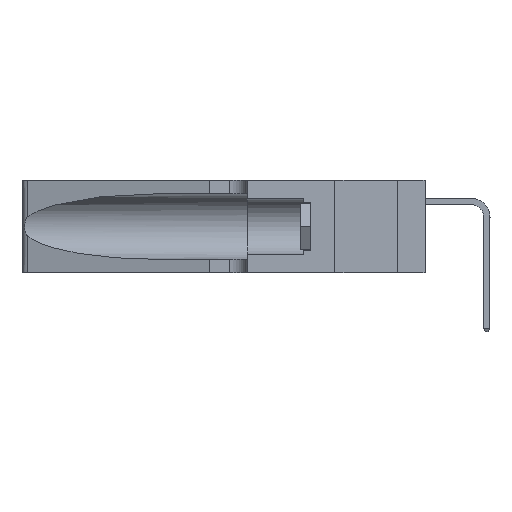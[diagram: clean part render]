
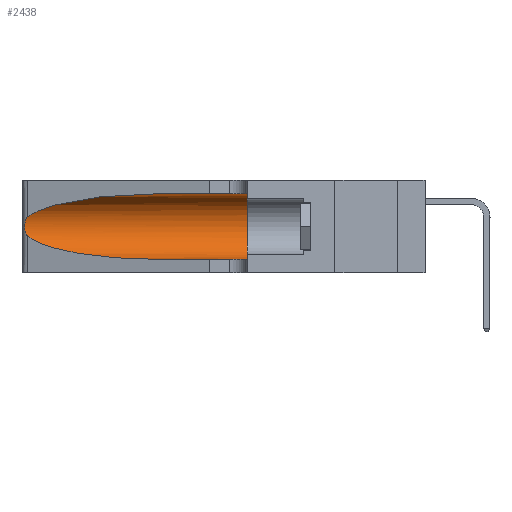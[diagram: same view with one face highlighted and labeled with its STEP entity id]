
A CAD part, left-side view. The second image highlights one B-rep face of the part: STEP entity #2438.
In plain terms, the highlighted cylindrical face has radius 3.308 mm (diameter 6.617 mm), a partial arc.
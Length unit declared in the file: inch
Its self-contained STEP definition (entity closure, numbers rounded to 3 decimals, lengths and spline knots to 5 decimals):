
#8 = CARTESIAN_POINT ( 'NONE',  ( 0.25854, 1.2359, 0.20912 ) ) ;
#1064 = CARTESIAN_POINT ( 'NONE',  ( 0.2373, 1.15595, 0.08982 ) ) ;
#1563 = AXIS2_PLACEMENT_3D ( 'NONE', #12583, #29313, #32099 ) ;
#2438 = ADVANCED_FACE ( 'NONE', ( #8639 ), #29799, .F. ) ;
#2806 = CARTESIAN_POINT ( 'NONE',  ( 0.26075, 1.23896, 0.19203 ) ) ;
#3381 = VERTEX_POINT ( 'NONE', #5818 ) ;
#3689 =( BOUNDED_CURVE ( )  B_SPLINE_CURVE ( 3, ( #4018, #1064, #9629, #28894 ),
 .UNSPECIFIED., .F., .T. ) 
 B_SPLINE_CURVE_WITH_KNOTS ( ( 4, 4 ),
 ( 3.44316, 4.71239 ),
 .UNSPECIFIED. ) 
 CURVE ( )  GEOMETRIC_REPRESENTATION_ITEM ( )  RATIONAL_B_SPLINE_CURVE ( ( 1., 0.87, 0.87, 1. ) ) 
 REPRESENTATION_ITEM ( '' )  );
#4018 = CARTESIAN_POINT ( 'NONE',  ( 0.25487, 1.22718, 0.14631 ) ) ;
#4742 = CARTESIAN_POINT ( 'NONE',  ( 0.1305, 1.61858, 0.05475 ) ) ;
#4888 = DIRECTION ( 'NONE',  ( 0., 1., 0. ) ) ;
#5633 = CARTESIAN_POINT ( 'NONE',  ( 0.26017, 1.23833, 0.17102 ) ) ;
#5818 = CARTESIAN_POINT ( 'NONE',  ( 0.1305, 0.72297, 0.05475 ) ) ;
#6177 = EDGE_CURVE ( 'NONE', #21253, #7064, #14655, .T. ) ;
#7064 = VERTEX_POINT ( 'NONE', #15057 ) ;
#7546 = DIRECTION ( 'NONE',  ( 0., -1., 0. ) ) ;
#7639 =( BOUNDED_CURVE ( )  B_SPLINE_CURVE ( 3, ( #24310, #21574, #27076, #10600 ),
 .UNSPECIFIED., .F., .F. ) 
 B_SPLINE_CURVE_WITH_KNOTS ( ( 4, 4 ),
 ( 1.5708, 2.84003 ),
 .UNSPECIFIED. ) 
 CURVE ( )  GEOMETRIC_REPRESENTATION_ITEM ( )  RATIONAL_B_SPLINE_CURVE ( ( 1., 0.87, 0.87, 1. ) ) 
 REPRESENTATION_ITEM ( '' )  );
#8177 = ORIENTED_EDGE ( 'NONE', *, *, #16477, .F. ) ;
#8419 = CARTESIAN_POINT ( 'NONE',  ( 0.25789, 1.23486, 0.15765 ) ) ;
#8639 = FACE_OUTER_BOUND ( 'NONE', #27066, .T. ) ;
#9629 = CARTESIAN_POINT ( 'NONE',  ( 0.18966, 0.96281, 0.05475 ) ) ;
#10600 = CARTESIAN_POINT ( 'NONE',  ( 0.25487, 1.22718, 0.22369 ) ) ;
#11242 = CARTESIAN_POINT ( 'NONE',  ( 0.25555, 1.22993, 0.14849 ) ) ;
#11387 = LINE ( 'NONE', #17877, #26026 ) ;
#11479 = ORIENTED_EDGE ( 'NONE', *, *, #28971, .F. ) ;
#11664 = CIRCLE ( 'NONE', #32543, 0.13025 ) ;
#12299 = DIRECTION ( 'NONE',  ( 0., -1., 0. ) ) ;
#12412 = VERTEX_POINT ( 'NONE', #30438 ) ;
#12583 = CARTESIAN_POINT ( 'NONE',  ( 0.1305, 1.61858, 0.185 ) ) ;
#14443 = LINE ( 'NONE', #4742, #21765 ) ;
#14655 = B_SPLINE_CURVE_WITH_KNOTS ( 'NONE', 3,
 ( #33154, #24846, #27598, #16706, #8, #19470, #2806, #22219, #5633, #24971, #8419, #27720, #11242, #30504 ),
 .UNSPECIFIED., .F., .F.,
 ( 4, 2, 2, 2, 2, 2, 4 ),
 ( 0., 0.00027, 0.00053, 0.00107, 0.0016, 0.00187, 0.00214 ),
 .UNSPECIFIED. ) ;
#15057 = CARTESIAN_POINT ( 'NONE',  ( 0.25487, 1.22718, 0.14631 ) ) ;
#16420 = CARTESIAN_POINT ( 'NONE',  ( 0.25487, 1.22718, 0.22369 ) ) ;
#16477 = EDGE_CURVE ( 'NONE', #31257, #26267, #11664, .T. ) ;
#16706 = CARTESIAN_POINT ( 'NONE',  ( 0.25787, 1.23484, 0.2124 ) ) ;
#17877 = CARTESIAN_POINT ( 'NONE',  ( 0.1305, 1.61858, 0.31525 ) ) ;
#19073 = ORIENTED_EDGE ( 'NONE', *, *, #21090, .T. ) ;
#19214 = EDGE_CURVE ( 'NONE', #12412, #21253, #7639, .T. ) ;
#19470 = CARTESIAN_POINT ( 'NONE',  ( 0.26018, 1.23835, 0.19895 ) ) ;
#20655 = ORIENTED_EDGE ( 'NONE', *, *, #28978, .T. ) ;
#21090 = EDGE_CURVE ( 'NONE', #3381, #26267, #14443, .T. ) ;
#21253 = VERTEX_POINT ( 'NONE', #16420 ) ;
#21502 = CARTESIAN_POINT ( 'NONE',  ( 0.1305, 0.35, 0.185 ) ) ;
#21574 = CARTESIAN_POINT ( 'NONE',  ( 0.18966, 0.96281, 0.31525 ) ) ;
#21765 = VECTOR ( 'NONE', #7546, 39.37008 ) ;
#22219 = CARTESIAN_POINT ( 'NONE',  ( 0.26075, 1.23896, 0.178 ) ) ;
#24229 = DIRECTION ( 'NONE',  ( 0., 0., 1. ) ) ;
#24310 = CARTESIAN_POINT ( 'NONE',  ( 0.1305, 0.72297, 0.31525 ) ) ;
#24846 = CARTESIAN_POINT ( 'NONE',  ( 0.25555, 1.22994, 0.2215 ) ) ;
#24971 = CARTESIAN_POINT ( 'NONE',  ( 0.25856, 1.23593, 0.16098 ) ) ;
#26026 = VECTOR ( 'NONE', #12299, 39.37008 ) ;
#26267 = VERTEX_POINT ( 'NONE', #27997 ) ;
#26409 = ORIENTED_EDGE ( 'NONE', *, *, #19214, .T. ) ;
#27066 = EDGE_LOOP ( 'NONE', ( #26409, #32947, #20655, #19073, #8177, #11479 ) ) ;
#27076 = CARTESIAN_POINT ( 'NONE',  ( 0.2373, 1.15595, 0.28018 ) ) ;
#27598 = CARTESIAN_POINT ( 'NONE',  ( 0.25639, 1.23184, 0.21858 ) ) ;
#27720 = CARTESIAN_POINT ( 'NONE',  ( 0.25639, 1.23186, 0.15144 ) ) ;
#27908 = CARTESIAN_POINT ( 'NONE',  ( 0.1305, 0.35, 0.31525 ) ) ;
#27997 = CARTESIAN_POINT ( 'NONE',  ( 0.1305, 0.35, 0.05475 ) ) ;
#28894 = CARTESIAN_POINT ( 'NONE',  ( 0.1305, 0.72297, 0.05475 ) ) ;
#28971 = EDGE_CURVE ( 'NONE', #12412, #31257, #11387, .T. ) ;
#28978 = EDGE_CURVE ( 'NONE', #7064, #3381, #3689, .T. ) ;
#29313 = DIRECTION ( 'NONE',  ( 0., -1., 0. ) ) ;
#29799 = CYLINDRICAL_SURFACE ( 'NONE', #1563, 0.13025 ) ;
#30438 = CARTESIAN_POINT ( 'NONE',  ( 0.1305, 0.72297, 0.31525 ) ) ;
#30504 = CARTESIAN_POINT ( 'NONE',  ( 0.25487, 1.22718, 0.14631 ) ) ;
#31257 = VERTEX_POINT ( 'NONE', #27908 ) ;
#32099 = DIRECTION ( 'NONE',  ( 0., 0., -1. ) ) ;
#32543 = AXIS2_PLACEMENT_3D ( 'NONE', #21502, #4888, #24229 ) ;
#32947 = ORIENTED_EDGE ( 'NONE', *, *, #6177, .T. ) ;
#33154 = CARTESIAN_POINT ( 'NONE',  ( 0.25487, 1.22718, 0.22369 ) ) ;
